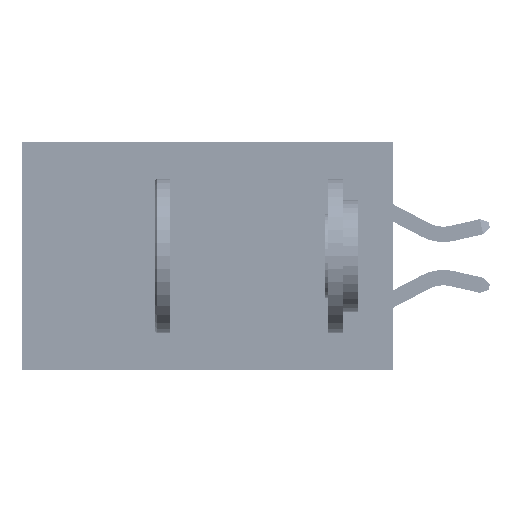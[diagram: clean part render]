
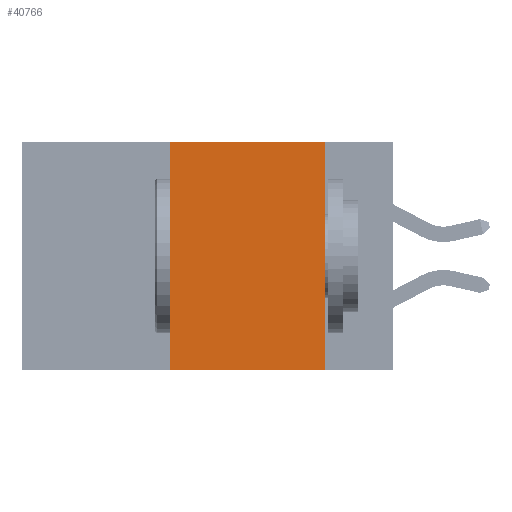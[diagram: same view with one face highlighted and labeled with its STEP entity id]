
A CAD part, left-side view. The second image highlights one B-rep face of the part: STEP entity #40766.
In plain terms, the highlighted planar face has unit normal (-1, 0, 0).
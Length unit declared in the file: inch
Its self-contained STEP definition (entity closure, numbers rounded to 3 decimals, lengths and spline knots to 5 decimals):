
#651 = VERTEX_POINT ( 'NONE', #22685 ) ;
#826 = DIRECTION ( 'NONE',  ( 0., -1., 0. ) ) ;
#1109 = ORIENTED_EDGE ( 'NONE', *, *, #37299, .F. ) ;
#3867 = CARTESIAN_POINT ( 'NONE',  ( 0., 0.11, 0. ) ) ;
#4381 = LINE ( 'NONE', #14529, #31720 ) ;
#5193 = ORIENTED_EDGE ( 'NONE', *, *, #12424, .T. ) ;
#5378 = LINE ( 'NONE', #27335, #18827 ) ;
#6198 = LINE ( 'NONE', #11304, #24961 ) ;
#6692 = DIRECTION ( 'NONE',  ( 0., -1., 0. ) ) ;
#7531 = PLANE ( 'NONE',  #28995 ) ;
#7680 = DIRECTION ( 'NONE',  ( 0., 0., 1. ) ) ;
#11304 = CARTESIAN_POINT ( 'NONE',  ( 0., 0.11, 0. ) ) ;
#12320 = ORIENTED_EDGE ( 'NONE', *, *, #13567, .F. ) ;
#12424 = EDGE_CURVE ( 'NONE', #34451, #651, #4381, .T. ) ;
#13217 = LINE ( 'NONE', #35199, #35684 ) ;
#13567 = EDGE_CURVE ( 'NONE', #31234, #27067, #5378, .T. ) ;
#14529 = CARTESIAN_POINT ( 'NONE',  ( 0., 0.6, -0.37 ) ) ;
#18018 = DIRECTION ( 'NONE',  ( 0., 0., -1. ) ) ;
#18827 = VECTOR ( 'NONE', #6692, 39.37008 ) ;
#22685 = CARTESIAN_POINT ( 'NONE',  ( 0., 0.11, -0.37 ) ) ;
#23591 = CARTESIAN_POINT ( 'NONE',  ( 0., 0.36, -0.37 ) ) ;
#24448 = DIRECTION ( 'NONE',  ( 1., 0., 0. ) ) ;
#24961 = VECTOR ( 'NONE', #41982, 39.37008 ) ;
#26454 = EDGE_CURVE ( 'NONE', #34451, #31234, #13217, .T. ) ;
#27067 = VERTEX_POINT ( 'NONE', #3867 ) ;
#27335 = CARTESIAN_POINT ( 'NONE',  ( 0., 0.6, 0. ) ) ;
#27770 = ORIENTED_EDGE ( 'NONE', *, *, #26454, .F. ) ;
#28993 = FACE_OUTER_BOUND ( 'NONE', #34828, .T. ) ;
#28995 = AXIS2_PLACEMENT_3D ( 'NONE', #38512, #24448, #18018 ) ;
#31234 = VERTEX_POINT ( 'NONE', #42950 ) ;
#31720 = VECTOR ( 'NONE', #826, 39.37008 ) ;
#34451 = VERTEX_POINT ( 'NONE', #23591 ) ;
#34828 = EDGE_LOOP ( 'NONE', ( #1109, #12320, #27770, #5193 ) ) ;
#35199 = CARTESIAN_POINT ( 'NONE',  ( 0., 0.36, 0. ) ) ;
#35684 = VECTOR ( 'NONE', #7680, 39.37008 ) ;
#37299 = EDGE_CURVE ( 'NONE', #27067, #651, #6198, .T. ) ;
#38512 = CARTESIAN_POINT ( 'NONE',  ( 0., 0.6, 0. ) ) ;
#40766 = ADVANCED_FACE ( 'NONE', ( #28993 ), #7531, .F. ) ;
#41982 = DIRECTION ( 'NONE',  ( 0., 0., -1. ) ) ;
#42950 = CARTESIAN_POINT ( 'NONE',  ( 0., 0.36, 0. ) ) ;
